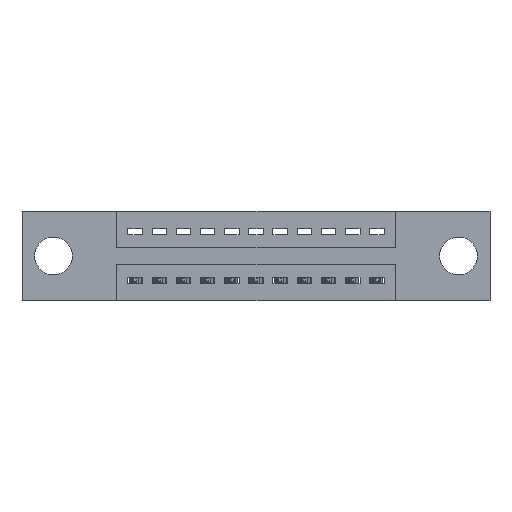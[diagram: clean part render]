
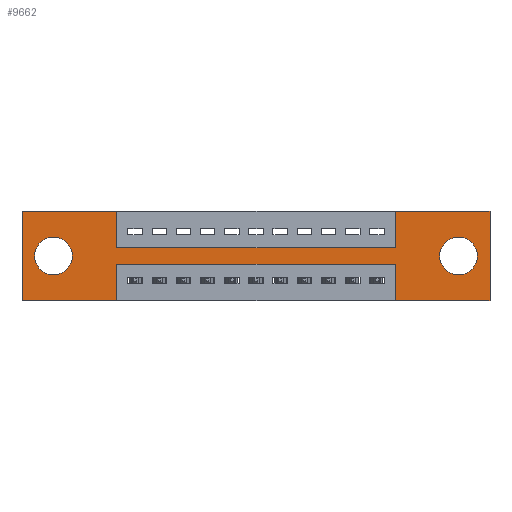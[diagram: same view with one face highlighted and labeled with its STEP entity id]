
A CAD part, front view. The second image highlights one B-rep face of the part: STEP entity #9662.
In plain terms, the highlighted planar face has unit normal (0, -1, 0).
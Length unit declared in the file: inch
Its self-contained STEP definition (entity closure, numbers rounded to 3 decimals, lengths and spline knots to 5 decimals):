
#368 = VERTEX_POINT ( 'NONE', #12232 ) ;
#486 = FACE_BOUND ( 'NONE', #10971, .T. ) ;
#720 = VERTEX_POINT ( 'NONE', #6405 ) ;
#804 = ORIENTED_EDGE ( 'NONE', *, *, #5410, .T. ) ;
#901 = CARTESIAN_POINT ( 'NONE',  ( 1.5425, 0., 0. ) ) ;
#1022 = CARTESIAN_POINT ( 'NONE',  ( 0., 0., -0.37 ) ) ;
#1061 = LINE ( 'NONE', #3587, #10423 ) ;
#1179 = DIRECTION ( 'NONE',  ( 0., 1., 0. ) ) ;
#1190 = CIRCLE ( 'NONE', #8402, 0.078 ) ;
#1307 = CARTESIAN_POINT ( 'NONE',  ( 1.805, 0., -0.185 ) ) ;
#1453 = ORIENTED_EDGE ( 'NONE', *, *, #7669, .F. ) ;
#1524 = CARTESIAN_POINT ( 'NONE',  ( 0.13, 0., -0.263 ) ) ;
#1606 = LINE ( 'NONE', #8244, #3441 ) ;
#1649 = CARTESIAN_POINT ( 'NONE',  ( 0., 0., 0. ) ) ;
#1701 = CARTESIAN_POINT ( 'NONE',  ( 1.935, 0., 0. ) ) ;
#1746 = CARTESIAN_POINT ( 'NONE',  ( 0.3925, 0., -0.22 ) ) ;
#1766 = CARTESIAN_POINT ( 'NONE',  ( 1.5425, 0., -0.15 ) ) ;
#1834 = LINE ( 'NONE', #2534, #11147 ) ;
#1870 = CARTESIAN_POINT ( 'NONE',  ( 0., 0., 0. ) ) ;
#1873 = EDGE_LOOP ( 'NONE', ( #2880, #5662 ) ) ;
#1966 = VECTOR ( 'NONE', #2679, 39.37008 ) ;
#2120 = EDGE_CURVE ( 'NONE', #7643, #7067, #2625, .T. ) ;
#2153 = ORIENTED_EDGE ( 'NONE', *, *, #7199, .T. ) ;
#2479 = AXIS2_PLACEMENT_3D ( 'NONE', #1307, #1179, #11828 ) ;
#2534 = CARTESIAN_POINT ( 'NONE',  ( 0., 0., -0.37 ) ) ;
#2625 = LINE ( 'NONE', #1870, #5927 ) ;
#2652 = DIRECTION ( 'NONE',  ( 0., 0., -1. ) ) ;
#2658 = LINE ( 'NONE', #1746, #8063 ) ;
#2679 = DIRECTION ( 'NONE',  ( 0., 0., -1. ) ) ;
#2704 = ORIENTED_EDGE ( 'NONE', *, *, #12165, .F. ) ;
#2738 = CARTESIAN_POINT ( 'NONE',  ( 0., 0., 0. ) ) ;
#2880 = ORIENTED_EDGE ( 'NONE', *, *, #5168, .T. ) ;
#3003 = VERTEX_POINT ( 'NONE', #8275 ) ;
#3337 = ORIENTED_EDGE ( 'NONE', *, *, #8365, .F. ) ;
#3406 = AXIS2_PLACEMENT_3D ( 'NONE', #11218, #7391, #3698 ) ;
#3441 = VECTOR ( 'NONE', #3467, 39.37008 ) ;
#3467 = DIRECTION ( 'NONE',  ( 0., 0., 1. ) ) ;
#3572 = EDGE_CURVE ( 'NONE', #7711, #4797, #1606, .T. ) ;
#3587 = CARTESIAN_POINT ( 'NONE',  ( 0.3925, 0., 0. ) ) ;
#3679 = DIRECTION ( 'NONE',  ( -1., 0., 0. ) ) ;
#3698 = DIRECTION ( 'NONE',  ( 0., 0., -1. ) ) ;
#3730 = EDGE_CURVE ( 'NONE', #368, #7643, #4813, .T. ) ;
#3806 = ORIENTED_EDGE ( 'NONE', *, *, #7397, .F. ) ;
#3855 = CARTESIAN_POINT ( 'NONE',  ( 0.13, 0., -0.185 ) ) ;
#3882 = CARTESIAN_POINT ( 'NONE',  ( 0.3925, 0., -0.15 ) ) ;
#4120 = EDGE_CURVE ( 'NONE', #7067, #11469, #9465, .T. ) ;
#4319 = LINE ( 'NONE', #7330, #10474 ) ;
#4345 = CARTESIAN_POINT ( 'NONE',  ( 0.3925, 0., -0.15 ) ) ;
#4356 = AXIS2_PLACEMENT_3D ( 'NONE', #3855, #4676, #8566 ) ;
#4466 = CIRCLE ( 'NONE', #4356, 0.078 ) ;
#4469 = CARTESIAN_POINT ( 'NONE',  ( 0.3925, 0., 0. ) ) ;
#4547 = CARTESIAN_POINT ( 'NONE',  ( 1.805, 0., -0.185 ) ) ;
#4556 = LINE ( 'NONE', #7728, #9377 ) ;
#4661 = VERTEX_POINT ( 'NONE', #10606 ) ;
#4676 = DIRECTION ( 'NONE',  ( 0., 1., 0. ) ) ;
#4797 = VERTEX_POINT ( 'NONE', #9627 ) ;
#4813 = LINE ( 'NONE', #1022, #12002 ) ;
#4895 = FACE_OUTER_BOUND ( 'NONE', #12304, .T. ) ;
#5168 = EDGE_CURVE ( 'NONE', #4661, #9593, #7757, .T. ) ;
#5329 = EDGE_CURVE ( 'NONE', #7836, #368, #4319, .T. ) ;
#5351 = VERTEX_POINT ( 'NONE', #1524 ) ;
#5410 = EDGE_CURVE ( 'NONE', #6636, #5351, #4466, .T. ) ;
#5449 = ORIENTED_EDGE ( 'NONE', *, *, #10411, .F. ) ;
#5467 = CARTESIAN_POINT ( 'NONE',  ( 0.3925, 0., -0.22 ) ) ;
#5662 = ORIENTED_EDGE ( 'NONE', *, *, #12173, .T. ) ;
#5927 = VECTOR ( 'NONE', #10543, 39.37008 ) ;
#6263 = VERTEX_POINT ( 'NONE', #4345 ) ;
#6376 = FACE_BOUND ( 'NONE', #1873, .T. ) ;
#6392 = DIRECTION ( 'NONE',  ( 1., 0., 0. ) ) ;
#6405 = CARTESIAN_POINT ( 'NONE',  ( 1.935, 0., -0.37 ) ) ;
#6625 = ORIENTED_EDGE ( 'NONE', *, *, #10121, .F. ) ;
#6636 = VERTEX_POINT ( 'NONE', #11917 ) ;
#6752 = ORIENTED_EDGE ( 'NONE', *, *, #4120, .F. ) ;
#6760 = DIRECTION ( 'NONE',  ( -1., 0., 0. ) ) ;
#6933 = CIRCLE ( 'NONE', #11750, 0.078 ) ;
#7059 = LINE ( 'NONE', #1701, #1966 ) ;
#7067 = VERTEX_POINT ( 'NONE', #2738 ) ;
#7199 = EDGE_CURVE ( 'NONE', #5351, #6636, #6933, .T. ) ;
#7330 = CARTESIAN_POINT ( 'NONE',  ( 0.3925, 0., -0.37 ) ) ;
#7358 = ORIENTED_EDGE ( 'NONE', *, *, #3572, .F. ) ;
#7391 = DIRECTION ( 'NONE',  ( 0., -1., 0. ) ) ;
#7397 = EDGE_CURVE ( 'NONE', #720, #7711, #1834, .T. ) ;
#7643 = VERTEX_POINT ( 'NONE', #8313 ) ;
#7669 = EDGE_CURVE ( 'NONE', #11469, #6263, #1061, .T. ) ;
#7711 = VERTEX_POINT ( 'NONE', #9868 ) ;
#7728 = CARTESIAN_POINT ( 'NONE',  ( 1.5425, 0., 0. ) ) ;
#7757 = CIRCLE ( 'NONE', #2479, 0.078 ) ;
#7801 = VERTEX_POINT ( 'NONE', #901 ) ;
#7836 = VERTEX_POINT ( 'NONE', #5467 ) ;
#7975 = CARTESIAN_POINT ( 'NONE',  ( 0.13, 0., -0.185 ) ) ;
#8063 = VECTOR ( 'NONE', #3679, 39.37008 ) ;
#8185 = LINE ( 'NONE', #3882, #11785 ) ;
#8244 = CARTESIAN_POINT ( 'NONE',  ( 1.5425, 0., -0.37 ) ) ;
#8275 = CARTESIAN_POINT ( 'NONE',  ( 1.935, 0., 0. ) ) ;
#8313 = CARTESIAN_POINT ( 'NONE',  ( 0., 0., -0.37 ) ) ;
#8365 = EDGE_CURVE ( 'NONE', #11846, #7801, #4556, .T. ) ;
#8402 = AXIS2_PLACEMENT_3D ( 'NONE', #4547, #12202, #11153 ) ;
#8475 = LINE ( 'NONE', #1649, #12066 ) ;
#8529 = DIRECTION ( 'NONE',  ( 1., 0., 0. ) ) ;
#8566 = DIRECTION ( 'NONE',  ( 0., 0., 1. ) ) ;
#8570 = CARTESIAN_POINT ( 'NONE',  ( 0., 0., 0. ) ) ;
#8708 = ORIENTED_EDGE ( 'NONE', *, *, #5329, .F. ) ;
#8955 = ORIENTED_EDGE ( 'NONE', *, *, #9056, .F. ) ;
#9056 = EDGE_CURVE ( 'NONE', #4797, #7836, #2658, .T. ) ;
#9186 = PLANE ( 'NONE',  #3406 ) ;
#9299 = DIRECTION ( 'NONE',  ( 0., 1., 0. ) ) ;
#9377 = VECTOR ( 'NONE', #10766, 39.37008 ) ;
#9465 = LINE ( 'NONE', #8570, #12138 ) ;
#9593 = VERTEX_POINT ( 'NONE', #10862 ) ;
#9627 = CARTESIAN_POINT ( 'NONE',  ( 1.5425, 0., -0.22 ) ) ;
#9662 = ADVANCED_FACE ( 'NONE', ( #6376, #486, #4895 ), #9186, .T. ) ;
#9868 = CARTESIAN_POINT ( 'NONE',  ( 1.5425, 0., -0.37 ) ) ;
#10121 = EDGE_CURVE ( 'NONE', #6263, #11846, #8185, .T. ) ;
#10411 = EDGE_CURVE ( 'NONE', #7801, #3003, #8475, .T. ) ;
#10423 = VECTOR ( 'NONE', #2652, 39.37008 ) ;
#10474 = VECTOR ( 'NONE', #12086, 39.37008 ) ;
#10543 = DIRECTION ( 'NONE',  ( 0., 0., 1. ) ) ;
#10606 = CARTESIAN_POINT ( 'NONE',  ( 1.805, 0., -0.107 ) ) ;
#10656 = DIRECTION ( 'NONE',  ( 1., 0., 0. ) ) ;
#10766 = DIRECTION ( 'NONE',  ( 0., 0., 1. ) ) ;
#10862 = CARTESIAN_POINT ( 'NONE',  ( 1.805, 0., -0.263 ) ) ;
#10908 = ORIENTED_EDGE ( 'NONE', *, *, #3730, .F. ) ;
#10971 = EDGE_LOOP ( 'NONE', ( #804, #2153 ) ) ;
#11147 = VECTOR ( 'NONE', #11222, 39.37008 ) ;
#11153 = DIRECTION ( 'NONE',  ( 0., 0., -1. ) ) ;
#11218 = CARTESIAN_POINT ( 'NONE',  ( 0., 0., -0.37 ) ) ;
#11222 = DIRECTION ( 'NONE',  ( -1., 0., 0. ) ) ;
#11410 = DIRECTION ( 'NONE',  ( 0., 0., 1. ) ) ;
#11469 = VERTEX_POINT ( 'NONE', #4469 ) ;
#11636 = ORIENTED_EDGE ( 'NONE', *, *, #2120, .F. ) ;
#11750 = AXIS2_PLACEMENT_3D ( 'NONE', #7975, #9299, #11410 ) ;
#11785 = VECTOR ( 'NONE', #10656, 39.37008 ) ;
#11828 = DIRECTION ( 'NONE',  ( 0., 0., -1. ) ) ;
#11846 = VERTEX_POINT ( 'NONE', #1766 ) ;
#11917 = CARTESIAN_POINT ( 'NONE',  ( 0.13, 0., -0.107 ) ) ;
#12002 = VECTOR ( 'NONE', #6760, 39.37008 ) ;
#12066 = VECTOR ( 'NONE', #6392, 39.37008 ) ;
#12086 = DIRECTION ( 'NONE',  ( 0., 0., -1. ) ) ;
#12138 = VECTOR ( 'NONE', #8529, 39.37008 ) ;
#12165 = EDGE_CURVE ( 'NONE', #3003, #720, #7059, .T. ) ;
#12173 = EDGE_CURVE ( 'NONE', #9593, #4661, #1190, .T. ) ;
#12202 = DIRECTION ( 'NONE',  ( 0., 1., 0. ) ) ;
#12232 = CARTESIAN_POINT ( 'NONE',  ( 0.3925, 0., -0.37 ) ) ;
#12304 = EDGE_LOOP ( 'NONE', ( #8708, #8955, #7358, #3806, #2704, #5449, #3337, #6625, #1453, #6752, #11636, #10908 ) ) ;
